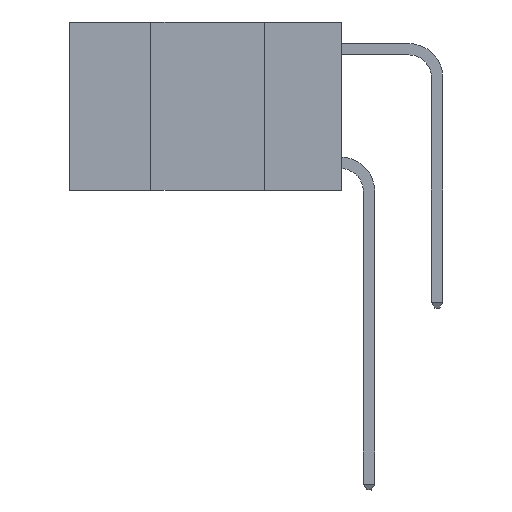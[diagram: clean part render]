
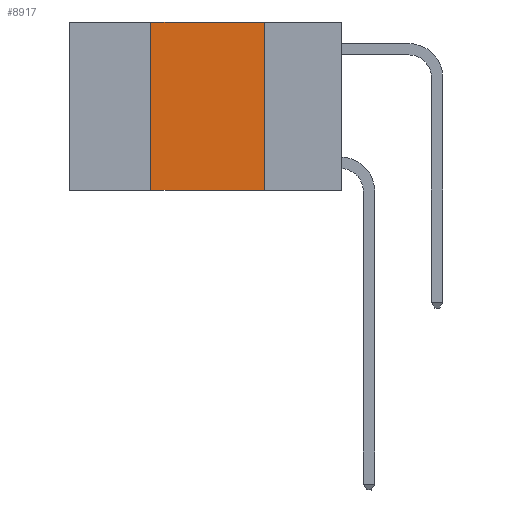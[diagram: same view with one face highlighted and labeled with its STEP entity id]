
A CAD part, left-side view. The second image highlights one B-rep face of the part: STEP entity #8917.
In plain terms, the highlighted planar face has unit normal (-1, 0, 0).
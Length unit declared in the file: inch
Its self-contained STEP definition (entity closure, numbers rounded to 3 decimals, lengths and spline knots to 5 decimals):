
#201 = EDGE_CURVE ( 'NONE', #10441, #2537, #3613, .T. ) ;
#1147 = CARTESIAN_POINT ( 'NONE',  ( 0., 0.17, 0. ) ) ;
#1684 = CARTESIAN_POINT ( 'NONE',  ( 0., 0.42, 0. ) ) ;
#2127 = ORIENTED_EDGE ( 'NONE', *, *, #11694, .F. ) ;
#2192 = ORIENTED_EDGE ( 'NONE', *, *, #12748, .F. ) ;
#2304 = DIRECTION ( 'NONE',  ( 0., 0., -1. ) ) ;
#2468 = ORIENTED_EDGE ( 'NONE', *, *, #8350, .F. ) ;
#2486 = ORIENTED_EDGE ( 'NONE', *, *, #201, .T. ) ;
#2537 = VERTEX_POINT ( 'NONE', #6827 ) ;
#2929 = DIRECTION ( 'NONE',  ( 1., 0., 0. ) ) ;
#3258 = DIRECTION ( 'NONE',  ( 0., -1., 0. ) ) ;
#3572 = LINE ( 'NONE', #6492, #11715 ) ;
#3613 = LINE ( 'NONE', #7254, #11747 ) ;
#4583 = VECTOR ( 'NONE', #11390, 39.37008 ) ;
#4654 = VERTEX_POINT ( 'NONE', #4959 ) ;
#4959 = CARTESIAN_POINT ( 'NONE',  ( 0., 0.17, 0. ) ) ;
#5084 = CARTESIAN_POINT ( 'NONE',  ( 0., 0.6, 0. ) ) ;
#5708 = FACE_OUTER_BOUND ( 'NONE', #8665, .T. ) ;
#6492 = CARTESIAN_POINT ( 'NONE',  ( 0., 0.6, 0. ) ) ;
#6827 = CARTESIAN_POINT ( 'NONE',  ( 0., 0.17, -0.37 ) ) ;
#7254 = CARTESIAN_POINT ( 'NONE',  ( 0., 0.6, -0.37 ) ) ;
#7402 = LINE ( 'NONE', #12490, #4583 ) ;
#8288 = VERTEX_POINT ( 'NONE', #1684 ) ;
#8350 = EDGE_CURVE ( 'NONE', #10441, #8288, #7402, .T. ) ;
#8665 = EDGE_LOOP ( 'NONE', ( #2127, #2192, #2468, #2486 ) ) ;
#8917 = ADVANCED_FACE ( 'NONE', ( #5708 ), #9364, .F. ) ;
#9119 = LINE ( 'NONE', #1147, #13964 ) ;
#9364 = PLANE ( 'NONE',  #10401 ) ;
#10401 = AXIS2_PLACEMENT_3D ( 'NONE', #5084, #2929, #10423 ) ;
#10423 = DIRECTION ( 'NONE',  ( 0., 0., -1. ) ) ;
#10441 = VERTEX_POINT ( 'NONE', #11795 ) ;
#11390 = DIRECTION ( 'NONE',  ( 0., 0., 1. ) ) ;
#11694 = EDGE_CURVE ( 'NONE', #4654, #2537, #9119, .T. ) ;
#11715 = VECTOR ( 'NONE', #3258, 39.37008 ) ;
#11747 = VECTOR ( 'NONE', #13524, 39.37008 ) ;
#11795 = CARTESIAN_POINT ( 'NONE',  ( 0., 0.42, -0.37 ) ) ;
#12490 = CARTESIAN_POINT ( 'NONE',  ( 0., 0.42, 0. ) ) ;
#12748 = EDGE_CURVE ( 'NONE', #8288, #4654, #3572, .T. ) ;
#13524 = DIRECTION ( 'NONE',  ( 0., -1., 0. ) ) ;
#13964 = VECTOR ( 'NONE', #2304, 39.37008 ) ;
